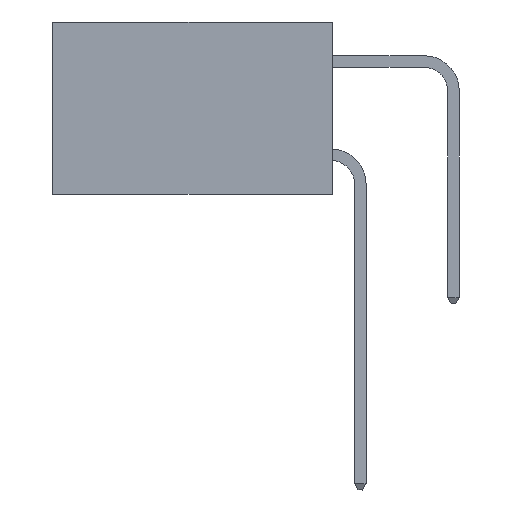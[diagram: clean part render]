
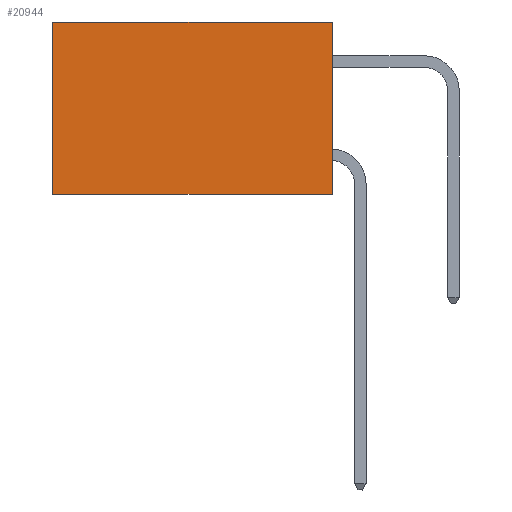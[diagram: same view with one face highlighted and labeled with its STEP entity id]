
A CAD part, left-side view. The second image highlights one B-rep face of the part: STEP entity #20944.
In plain terms, the highlighted planar face has unit normal (-1, 0, 0).
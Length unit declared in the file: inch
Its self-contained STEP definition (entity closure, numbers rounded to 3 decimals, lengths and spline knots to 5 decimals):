
#1972 = DIRECTION ( 'NONE',  ( 0., 1., 0. ) ) ;
#2092 = EDGE_LOOP ( 'NONE', ( #19928, #20621, #13390, #20356 ) ) ;
#2343 = DIRECTION ( 'NONE',  ( 0., 0., -1. ) ) ;
#3556 = DIRECTION ( 'NONE',  ( 0., 0., -1. ) ) ;
#4010 = DIRECTION ( 'NONE',  ( 0., 1., 0. ) ) ;
#7145 = CARTESIAN_POINT ( 'NONE',  ( 0.298, 0., -0.37 ) ) ;
#8705 = VECTOR ( 'NONE', #3556, 39.37008 ) ;
#8739 = CARTESIAN_POINT ( 'NONE',  ( 0.298, 0., 0. ) ) ;
#10152 = CARTESIAN_POINT ( 'NONE',  ( 0.298, 0.6, -0.37 ) ) ;
#10835 = EDGE_CURVE ( 'NONE', #32471, #33682, #29977, .T. ) ;
#11493 = CARTESIAN_POINT ( 'NONE',  ( 0.298, 0., 0. ) ) ;
#13390 = ORIENTED_EDGE ( 'NONE', *, *, #33421, .F. ) ;
#13657 = VECTOR ( 'NONE', #1972, 39.37008 ) ;
#14483 = LINE ( 'NONE', #8739, #8705 ) ;
#14489 = LINE ( 'NONE', #7145, #13657 ) ;
#16643 = CARTESIAN_POINT ( 'NONE',  ( 0.298, 0.6, 0. ) ) ;
#16915 = EDGE_CURVE ( 'NONE', #23890, #27886, #14489, .T. ) ;
#18105 = CARTESIAN_POINT ( 'NONE',  ( 0.298, 0.6, 0. ) ) ;
#18114 = CARTESIAN_POINT ( 'NONE',  ( 0.298, 0., 0. ) ) ;
#18674 = FACE_OUTER_BOUND ( 'NONE', #2092, .T. ) ;
#19928 = ORIENTED_EDGE ( 'NONE', *, *, #25218, .T. ) ;
#20356 = ORIENTED_EDGE ( 'NONE', *, *, #10835, .T. ) ;
#20427 = DIRECTION ( 'NONE',  ( 0., 0., -1. ) ) ;
#20621 = ORIENTED_EDGE ( 'NONE', *, *, #16915, .F. ) ;
#20768 = DIRECTION ( 'NONE',  ( 1., 0., 0. ) ) ;
#20847 = AXIS2_PLACEMENT_3D ( 'NONE', #30748, #20768, #20427 ) ;
#20944 = ADVANCED_FACE ( 'NONE', ( #18674 ), #28370, .F. ) ;
#22790 = CARTESIAN_POINT ( 'NONE',  ( 0.298, 0., -0.37 ) ) ;
#23890 = VERTEX_POINT ( 'NONE', #22790 ) ;
#25218 = EDGE_CURVE ( 'NONE', #33682, #27886, #28820, .T. ) ;
#27172 = VECTOR ( 'NONE', #2343, 39.37008 ) ;
#27886 = VERTEX_POINT ( 'NONE', #10152 ) ;
#28333 = VECTOR ( 'NONE', #4010, 39.37008 ) ;
#28370 = PLANE ( 'NONE',  #20847 ) ;
#28820 = LINE ( 'NONE', #18105, #27172 ) ;
#29977 = LINE ( 'NONE', #11493, #28333 ) ;
#30748 = CARTESIAN_POINT ( 'NONE',  ( 0.298, 0., 0. ) ) ;
#32471 = VERTEX_POINT ( 'NONE', #18114 ) ;
#33421 = EDGE_CURVE ( 'NONE', #32471, #23890, #14483, .T. ) ;
#33682 = VERTEX_POINT ( 'NONE', #16643 ) ;
